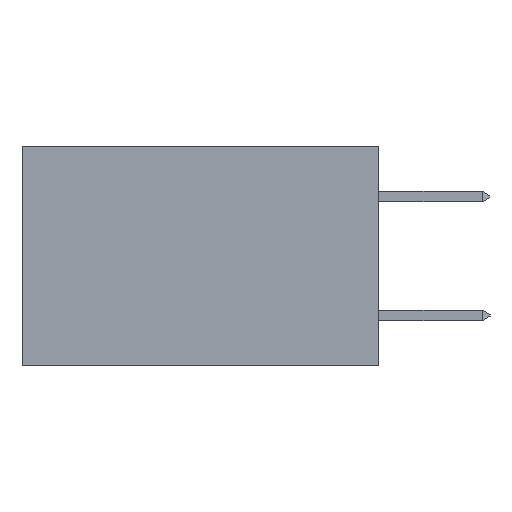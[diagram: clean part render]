
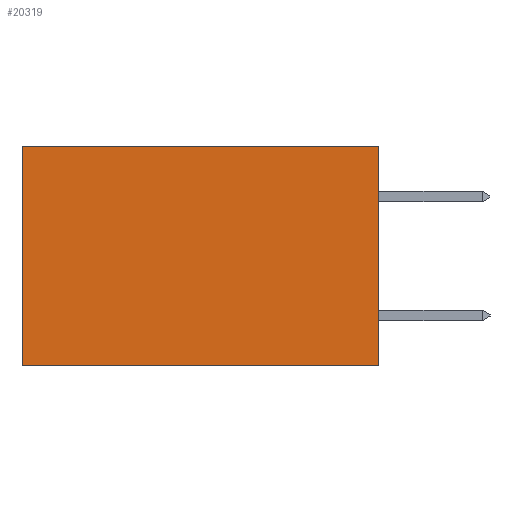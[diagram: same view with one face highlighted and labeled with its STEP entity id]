
A CAD part, left-side view. The second image highlights one B-rep face of the part: STEP entity #20319.
In plain terms, the highlighted planar face has unit normal (-1, 0, 0).
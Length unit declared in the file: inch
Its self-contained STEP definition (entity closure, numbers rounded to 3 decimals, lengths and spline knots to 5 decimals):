
#681 = DIRECTION ( 'NONE',  ( 1., 0., 0. ) ) ;
#892 = LINE ( 'NONE', #2482, #10413 ) ;
#2092 = VECTOR ( 'NONE', #23457, 39.37008 ) ;
#2482 = CARTESIAN_POINT ( 'NONE',  ( 0.2615, 0., 0. ) ) ;
#4428 = CARTESIAN_POINT ( 'NONE',  ( 0.2615, 0., -0.37 ) ) ;
#4557 = EDGE_CURVE ( 'NONE', #23865, #12082, #23109, .T. ) ;
#4656 = EDGE_CURVE ( 'NONE', #23865, #5434, #892, .T. ) ;
#5434 = VERTEX_POINT ( 'NONE', #12425 ) ;
#6363 = LINE ( 'NONE', #14069, #11488 ) ;
#7562 = ORIENTED_EDGE ( 'NONE', *, *, #4656, .T. ) ;
#7745 = CARTESIAN_POINT ( 'NONE',  ( 0.2615, 0., -0.37 ) ) ;
#9341 = DIRECTION ( 'NONE',  ( 0., 1., 0. ) ) ;
#9687 = EDGE_CURVE ( 'NONE', #12082, #23701, #12008, .T. ) ;
#10179 = DIRECTION ( 'NONE',  ( 0., 0., -1. ) ) ;
#10413 = VECTOR ( 'NONE', #9341, 39.37008 ) ;
#11488 = VECTOR ( 'NONE', #10179, 39.37008 ) ;
#12008 = LINE ( 'NONE', #14521, #21680 ) ;
#12082 = VERTEX_POINT ( 'NONE', #4428 ) ;
#12106 = CARTESIAN_POINT ( 'NONE',  ( 0.2615, 0., -0.37 ) ) ;
#12425 = CARTESIAN_POINT ( 'NONE',  ( 0.2615, 0.6, 0. ) ) ;
#12751 = FACE_OUTER_BOUND ( 'NONE', #24490, .T. ) ;
#13472 = CARTESIAN_POINT ( 'NONE',  ( 0.2615, 0.6, -0.37 ) ) ;
#14043 = DIRECTION ( 'NONE',  ( 0., 0., -1. ) ) ;
#14069 = CARTESIAN_POINT ( 'NONE',  ( 0.2615, 0.6, -0.37 ) ) ;
#14399 = ORIENTED_EDGE ( 'NONE', *, *, #21730, .T. ) ;
#14432 = DIRECTION ( 'NONE',  ( 0., 1., 0. ) ) ;
#14521 = CARTESIAN_POINT ( 'NONE',  ( 0.2615, 0., -0.37 ) ) ;
#14545 = AXIS2_PLACEMENT_3D ( 'NONE', #12106, #681, #14043 ) ;
#17864 = PLANE ( 'NONE',  #14545 ) ;
#20155 = CARTESIAN_POINT ( 'NONE',  ( 0.2615, 0., 0. ) ) ;
#20319 = ADVANCED_FACE ( 'NONE', ( #12751 ), #17864, .F. ) ;
#20907 = ORIENTED_EDGE ( 'NONE', *, *, #4557, .F. ) ;
#21680 = VECTOR ( 'NONE', #14432, 39.37008 ) ;
#21730 = EDGE_CURVE ( 'NONE', #5434, #23701, #6363, .T. ) ;
#23092 = ORIENTED_EDGE ( 'NONE', *, *, #9687, .F. ) ;
#23109 = LINE ( 'NONE', #7745, #2092 ) ;
#23457 = DIRECTION ( 'NONE',  ( 0., 0., -1. ) ) ;
#23701 = VERTEX_POINT ( 'NONE', #13472 ) ;
#23865 = VERTEX_POINT ( 'NONE', #20155 ) ;
#24490 = EDGE_LOOP ( 'NONE', ( #14399, #23092, #20907, #7562 ) ) ;
